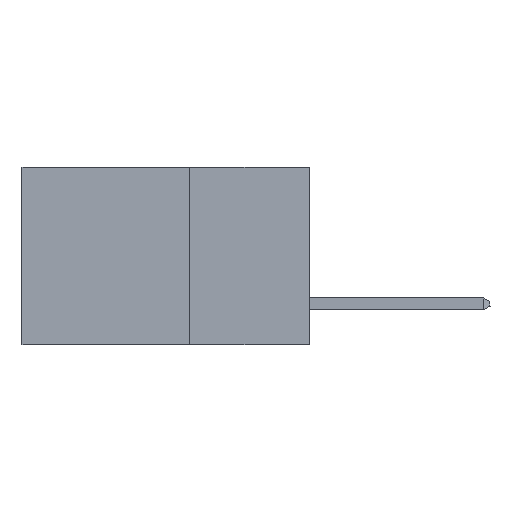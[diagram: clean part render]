
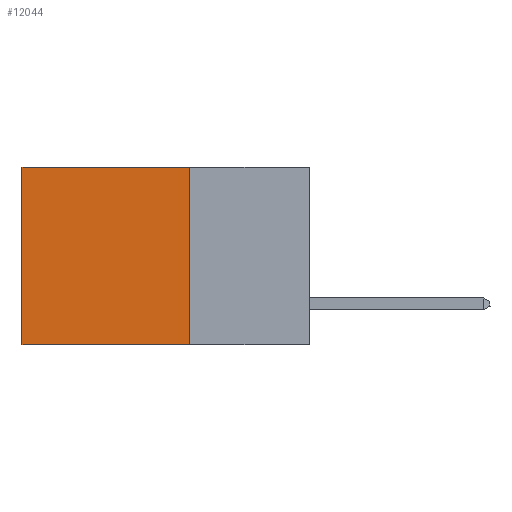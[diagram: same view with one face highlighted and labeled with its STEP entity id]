
A CAD part, left-side view. The second image highlights one B-rep face of the part: STEP entity #12044.
In plain terms, the highlighted planar face has unit normal (-1, 0, 0).
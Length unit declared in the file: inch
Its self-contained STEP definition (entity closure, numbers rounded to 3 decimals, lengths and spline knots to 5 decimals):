
#2939 = CARTESIAN_POINT ( 'NONE',  ( 0.2875, 0.6, 0. ) ) ;
#3249 = FACE_OUTER_BOUND ( 'NONE', #15750, .T. ) ;
#3657 = VERTEX_POINT ( 'NONE', #13034 ) ;
#3814 = VERTEX_POINT ( 'NONE', #13796 ) ;
#4372 = PLANE ( 'NONE',  #18436 ) ;
#5267 = DIRECTION ( 'NONE',  ( 0., 0., -1. ) ) ;
#5331 = DIRECTION ( 'NONE',  ( 0., 0., -1. ) ) ;
#5566 = ORIENTED_EDGE ( 'NONE', *, *, #8197, .T. ) ;
#6421 = VECTOR ( 'NONE', #10130, 39.37008 ) ;
#6466 = VECTOR ( 'NONE', #14287, 39.37008 ) ;
#6634 = ORIENTED_EDGE ( 'NONE', *, *, #26944, .F. ) ;
#7934 = ORIENTED_EDGE ( 'NONE', *, *, #25070, .T. ) ;
#8197 = EDGE_CURVE ( 'NONE', #18796, #3814, #17995, .T. ) ;
#8912 = DIRECTION ( 'NONE',  ( 1., 0., 0. ) ) ;
#10130 = DIRECTION ( 'NONE',  ( 0., 1., 0. ) ) ;
#10334 = CARTESIAN_POINT ( 'NONE',  ( 0.2875, 0.6, 0. ) ) ;
#12044 = ADVANCED_FACE ( 'NONE', ( #3249 ), #4372, .F. ) ;
#12406 = CARTESIAN_POINT ( 'NONE',  ( 0.2875, 0.25, -0.37 ) ) ;
#13034 = CARTESIAN_POINT ( 'NONE',  ( 0.2875, 0.25, -0.37 ) ) ;
#13796 = CARTESIAN_POINT ( 'NONE',  ( 0.2875, 0.6, -0.37 ) ) ;
#14287 = DIRECTION ( 'NONE',  ( 0., 1., 0. ) ) ;
#15750 = EDGE_LOOP ( 'NONE', ( #5566, #6634, #15769, #7934 ) ) ;
#15769 = ORIENTED_EDGE ( 'NONE', *, *, #28706, .F. ) ;
#17995 = LINE ( 'NONE', #2939, #28909 ) ;
#18436 = AXIS2_PLACEMENT_3D ( 'NONE', #22002, #8912, #20065 ) ;
#18796 = VERTEX_POINT ( 'NONE', #10334 ) ;
#19021 = LINE ( 'NONE', #20753, #21135 ) ;
#19550 = VERTEX_POINT ( 'NONE', #21069 ) ;
#20065 = DIRECTION ( 'NONE',  ( 0., 0., -1. ) ) ;
#20753 = CARTESIAN_POINT ( 'NONE',  ( 0.2875, 0.25, 0. ) ) ;
#21069 = CARTESIAN_POINT ( 'NONE',  ( 0.2875, 0.25, 0. ) ) ;
#21135 = VECTOR ( 'NONE', #5267, 39.37008 ) ;
#21609 = LINE ( 'NONE', #23544, #6466 ) ;
#22002 = CARTESIAN_POINT ( 'NONE',  ( 0.2875, 0.25, 0. ) ) ;
#23544 = CARTESIAN_POINT ( 'NONE',  ( 0.2875, 0.25, 0. ) ) ;
#25070 = EDGE_CURVE ( 'NONE', #19550, #18796, #21609, .T. ) ;
#26483 = LINE ( 'NONE', #12406, #6421 ) ;
#26944 = EDGE_CURVE ( 'NONE', #3657, #3814, #26483, .T. ) ;
#28706 = EDGE_CURVE ( 'NONE', #19550, #3657, #19021, .T. ) ;
#28909 = VECTOR ( 'NONE', #5331, 39.37008 ) ;
